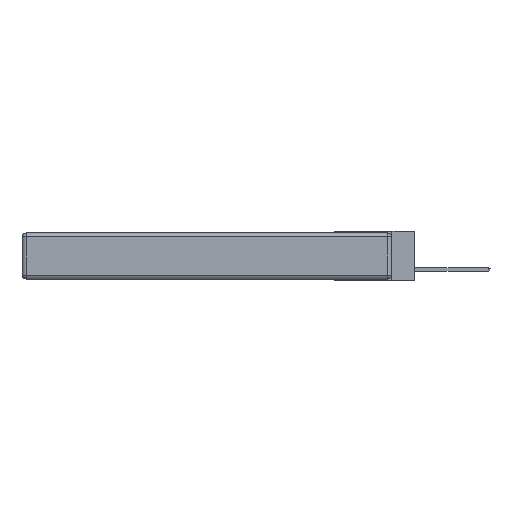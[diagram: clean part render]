
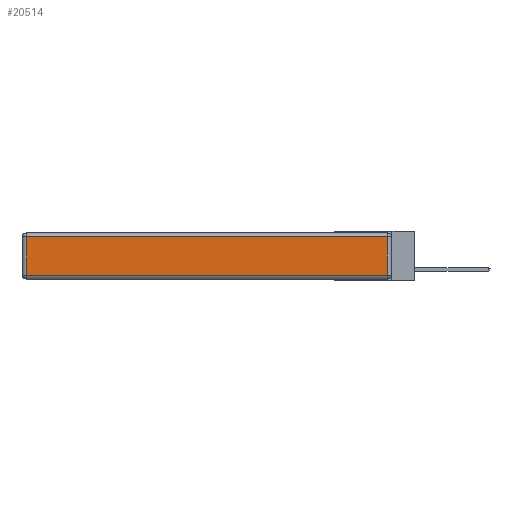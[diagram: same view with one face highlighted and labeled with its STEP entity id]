
A CAD part, left-side view. The second image highlights one B-rep face of the part: STEP entity #20514.
In plain terms, the highlighted planar face has unit normal (-1, 0, 0).
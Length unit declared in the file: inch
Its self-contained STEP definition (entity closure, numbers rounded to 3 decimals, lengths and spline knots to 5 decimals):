
#2255 = DIRECTION ( 'NONE',  ( 0., 0., 1. ) ) ;
#2289 = VERTEX_POINT ( 'NONE', #14741 ) ;
#2416 = CARTESIAN_POINT ( 'NONE',  ( 0., 0.03, -0.343 ) ) ;
#2445 = VERTEX_POINT ( 'NONE', #7043 ) ;
#2878 = EDGE_CURVE ( 'NONE', #2289, #20953, #4078, .T. ) ;
#3597 = ORIENTED_EDGE ( 'NONE', *, *, #12006, .T. ) ;
#4078 = LINE ( 'NONE', #2416, #24911 ) ;
#4180 = DIRECTION ( 'NONE',  ( 0., 0., 1. ) ) ;
#4534 = VECTOR ( 'NONE', #15053, 39.37008 ) ;
#5898 = CARTESIAN_POINT ( 'NONE',  ( 0., 2.72, -0.343 ) ) ;
#7043 = CARTESIAN_POINT ( 'NONE',  ( 0., 2.72, -0.03 ) ) ;
#8140 = DIRECTION ( 'NONE',  ( 0., -1., 0. ) ) ;
#8248 = DIRECTION ( 'NONE',  ( -1., 0., 0. ) ) ;
#8257 = ORIENTED_EDGE ( 'NONE', *, *, #16303, .T. ) ;
#9767 = DIRECTION ( 'NONE',  ( 0., 0., -1. ) ) ;
#9796 = EDGE_CURVE ( 'NONE', #23892, #2289, #17076, .T. ) ;
#9905 = PLANE ( 'NONE',  #11508 ) ;
#11508 = AXIS2_PLACEMENT_3D ( 'NONE', #22190, #8248, #4180 ) ;
#12006 = EDGE_CURVE ( 'NONE', #20953, #2445, #15289, .T. ) ;
#12167 = ORIENTED_EDGE ( 'NONE', *, *, #2878, .T. ) ;
#12539 = EDGE_LOOP ( 'NONE', ( #21901, #12167, #3597, #8257 ) ) ;
#12589 = VECTOR ( 'NONE', #8140, 39.37008 ) ;
#12609 = FACE_OUTER_BOUND ( 'NONE', #12539, .T. ) ;
#14741 = CARTESIAN_POINT ( 'NONE',  ( 0., 0.03, -0.313 ) ) ;
#15053 = DIRECTION ( 'NONE',  ( 0., 1., 0. ) ) ;
#15289 = LINE ( 'NONE', #24932, #4534 ) ;
#15999 = VECTOR ( 'NONE', #9767, 39.37008 ) ;
#16303 = EDGE_CURVE ( 'NONE', #2445, #23892, #22633, .T. ) ;
#16564 = CARTESIAN_POINT ( 'NONE',  ( 0., 2.72, -0.313 ) ) ;
#17076 = LINE ( 'NONE', #20216, #12589 ) ;
#18688 = CARTESIAN_POINT ( 'NONE',  ( 0., 0.03, -0.03 ) ) ;
#20216 = CARTESIAN_POINT ( 'NONE',  ( 0., 0., -0.313 ) ) ;
#20514 = ADVANCED_FACE ( 'NONE', ( #12609 ), #9905, .T. ) ;
#20953 = VERTEX_POINT ( 'NONE', #18688 ) ;
#21901 = ORIENTED_EDGE ( 'NONE', *, *, #9796, .T. ) ;
#22190 = CARTESIAN_POINT ( 'NONE',  ( 0., 0., -0.343 ) ) ;
#22633 = LINE ( 'NONE', #5898, #15999 ) ;
#23892 = VERTEX_POINT ( 'NONE', #16564 ) ;
#24911 = VECTOR ( 'NONE', #2255, 39.37008 ) ;
#24932 = CARTESIAN_POINT ( 'NONE',  ( 0., 2.75, -0.03 ) ) ;
